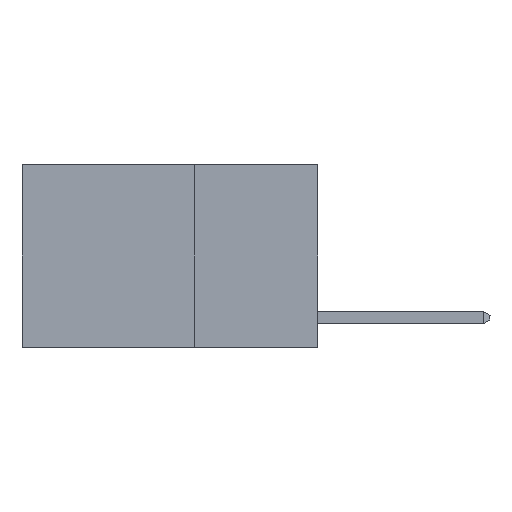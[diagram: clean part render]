
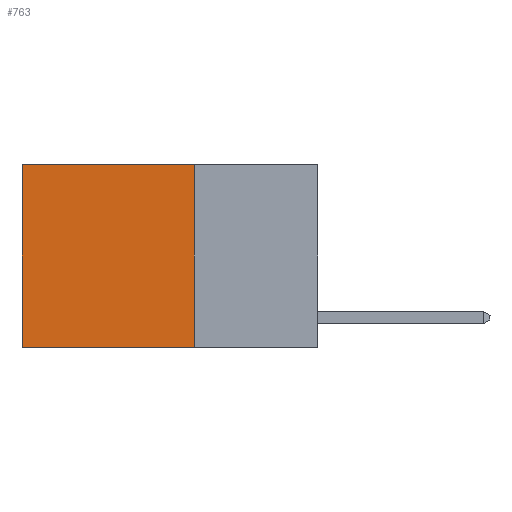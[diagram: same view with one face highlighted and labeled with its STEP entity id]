
A CAD part, left-side view. The second image highlights one B-rep face of the part: STEP entity #763.
In plain terms, the highlighted planar face has unit normal (-1, 0, 0).
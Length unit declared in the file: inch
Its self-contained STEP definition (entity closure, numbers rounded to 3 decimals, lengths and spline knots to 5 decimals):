
#261 = CARTESIAN_POINT ( 'NONE',  ( 0.2625, 0.6, -0.37 ) ) ;
#505 = ORIENTED_EDGE ( 'NONE', *, *, #1032, .F. ) ;
#763 = ADVANCED_FACE ( 'NONE', ( #10635 ), #12815, .F. ) ;
#1000 = CARTESIAN_POINT ( 'NONE',  ( 0.2625, 0.6, 0. ) ) ;
#1032 = EDGE_CURVE ( 'NONE', #8484, #11708, #7200, .T. ) ;
#1217 = DIRECTION ( 'NONE',  ( 1., 0., 0. ) ) ;
#1565 = AXIS2_PLACEMENT_3D ( 'NONE', #10691, #1217, #3294 ) ;
#2064 = LINE ( 'NONE', #1000, #9853 ) ;
#2848 = CARTESIAN_POINT ( 'NONE',  ( 0.2625, 0.25, 0. ) ) ;
#3045 = EDGE_CURVE ( 'NONE', #8484, #5744, #5954, .T. ) ;
#3294 = DIRECTION ( 'NONE',  ( 0., 0., -1. ) ) ;
#3792 = VECTOR ( 'NONE', #12536, 39.37008 ) ;
#4004 = CARTESIAN_POINT ( 'NONE',  ( 0.2625, 0.25, -0.37 ) ) ;
#4237 = DIRECTION ( 'NONE',  ( 0., 0., -1. ) ) ;
#4892 = CARTESIAN_POINT ( 'NONE',  ( 0.2625, 0.6, 0. ) ) ;
#5295 = VECTOR ( 'NONE', #11380, 39.37008 ) ;
#5744 = VERTEX_POINT ( 'NONE', #4892 ) ;
#5954 = LINE ( 'NONE', #12327, #5295 ) ;
#6176 = EDGE_LOOP ( 'NONE', ( #12846, #8302, #505, #8078 ) ) ;
#6319 = VECTOR ( 'NONE', #4237, 39.37008 ) ;
#6593 = CARTESIAN_POINT ( 'NONE',  ( 0.2625, 0.25, 0. ) ) ;
#7148 = VERTEX_POINT ( 'NONE', #261 ) ;
#7200 = LINE ( 'NONE', #2848, #6319 ) ;
#7849 = EDGE_CURVE ( 'NONE', #5744, #7148, #2064, .T. ) ;
#8078 = ORIENTED_EDGE ( 'NONE', *, *, #3045, .T. ) ;
#8302 = ORIENTED_EDGE ( 'NONE', *, *, #8402, .F. ) ;
#8402 = EDGE_CURVE ( 'NONE', #11708, #7148, #13589, .T. ) ;
#8484 = VERTEX_POINT ( 'NONE', #6593 ) ;
#8533 = DIRECTION ( 'NONE',  ( 0., 0., -1. ) ) ;
#8968 = CARTESIAN_POINT ( 'NONE',  ( 0.2625, 0.25, -0.37 ) ) ;
#9853 = VECTOR ( 'NONE', #8533, 39.37008 ) ;
#10635 = FACE_OUTER_BOUND ( 'NONE', #6176, .T. ) ;
#10691 = CARTESIAN_POINT ( 'NONE',  ( 0.2625, 0.25, 0. ) ) ;
#11380 = DIRECTION ( 'NONE',  ( 0., 1., 0. ) ) ;
#11708 = VERTEX_POINT ( 'NONE', #8968 ) ;
#12327 = CARTESIAN_POINT ( 'NONE',  ( 0.2625, 0.25, 0. ) ) ;
#12536 = DIRECTION ( 'NONE',  ( 0., 1., 0. ) ) ;
#12815 = PLANE ( 'NONE',  #1565 ) ;
#12846 = ORIENTED_EDGE ( 'NONE', *, *, #7849, .T. ) ;
#13589 = LINE ( 'NONE', #4004, #3792 ) ;
